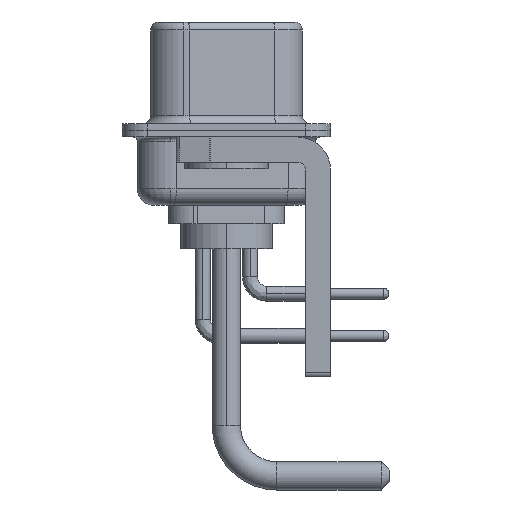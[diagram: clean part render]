
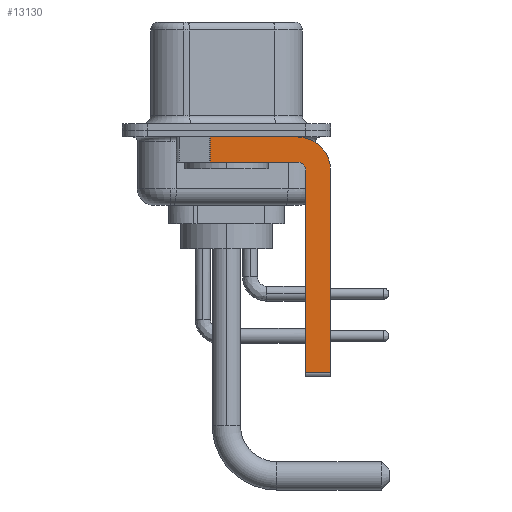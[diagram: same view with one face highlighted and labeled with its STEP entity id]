
A CAD part, left-side view. The second image highlights one B-rep face of the part: STEP entity #13130.
In plain terms, the highlighted planar face has unit normal (-1, 0, 0).
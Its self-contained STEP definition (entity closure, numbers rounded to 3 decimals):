
#246 = DIRECTION ( 'NONE',  ( 0., 0., -1. ) ) ;
#262 = EDGE_CURVE ( 'NONE', #14197, #24894, #24503, .T. ) ;
#716 = CARTESIAN_POINT ( 'NONE',  ( -2.9, -4.25, -2.4 ) ) ;
#851 = VERTEX_POINT ( 'NONE', #15234 ) ;
#991 = CIRCLE ( 'NONE', #23414, 0.5 ) ;
#1104 = CARTESIAN_POINT ( 'NONE',  ( -2.9, -4.25, -14.55 ) ) ;
#1154 = EDGE_CURVE ( 'NONE', #7924, #11928, #16393, .T. ) ;
#1262 = ORIENTED_EDGE ( 'NONE', *, *, #262, .F. ) ;
#1675 = CARTESIAN_POINT ( 'NONE',  ( -2.9, 0.978, -0.4 ) ) ;
#1800 = CIRCLE ( 'NONE', #5469, 2. ) ;
#2226 = CARTESIAN_POINT ( 'NONE',  ( -2.9, -4.25, -0.4 ) ) ;
#2501 = FACE_OUTER_BOUND ( 'NONE', #18995, .T. ) ;
#3681 = LINE ( 'NONE', #13634, #13141 ) ;
#4321 = DIRECTION ( 'NONE',  ( 1., 0., 0. ) ) ;
#4756 = CARTESIAN_POINT ( 'NONE',  ( -2.9, -6.25, -2.4 ) ) ;
#5011 = ORIENTED_EDGE ( 'NONE', *, *, #17259, .F. ) ;
#5469 = AXIS2_PLACEMENT_3D ( 'NONE', #20287, #4321, #18129 ) ;
#5486 = VERTEX_POINT ( 'NONE', #23102 ) ;
#5667 = CARTESIAN_POINT ( 'NONE',  ( -2.9, -4.25, -1.9 ) ) ;
#5718 = ORIENTED_EDGE ( 'NONE', *, *, #13471, .F. ) ;
#6594 = PLANE ( 'NONE',  #18527 ) ;
#7325 = VERTEX_POINT ( 'NONE', #8701 ) ;
#7575 = VERTEX_POINT ( 'NONE', #21443 ) ;
#7924 = VERTEX_POINT ( 'NONE', #23933 ) ;
#7932 = EDGE_CURVE ( 'NONE', #851, #7325, #12170, .T. ) ;
#8411 = VECTOR ( 'NONE', #23163, 1000. ) ;
#8622 = CARTESIAN_POINT ( 'NONE',  ( -2.9, -4.75, -14.8 ) ) ;
#8680 = DIRECTION ( 'NONE',  ( -1., 0., 0. ) ) ;
#8701 = CARTESIAN_POINT ( 'NONE',  ( -2.9, -4.75, -2.4 ) ) ;
#9018 = LINE ( 'NONE', #1104, #21106 ) ;
#9180 = ORIENTED_EDGE ( 'NONE', *, *, #10084, .T. ) ;
#9408 = VECTOR ( 'NONE', #16270, 1000. ) ;
#10084 = EDGE_CURVE ( 'NONE', #14197, #5486, #3681, .T. ) ;
#11452 = ORIENTED_EDGE ( 'NONE', *, *, #7932, .F. ) ;
#11636 = EDGE_CURVE ( 'NONE', #24894, #7924, #1800, .T. ) ;
#11928 = VERTEX_POINT ( 'NONE', #15655 ) ;
#12170 = LINE ( 'NONE', #8622, #9408 ) ;
#12856 = DIRECTION ( 'NONE',  ( 0., -1., 0. ) ) ;
#13126 = VECTOR ( 'NONE', #12856, 1000. ) ;
#13130 = ADVANCED_FACE ( 'NONE', ( #2501 ), #6594, .F. ) ;
#13141 = VECTOR ( 'NONE', #246, 1000. ) ;
#13471 = EDGE_CURVE ( 'NONE', #7575, #5486, #13690, .T. ) ;
#13634 = CARTESIAN_POINT ( 'NONE',  ( -2.9, 0.978, -1.9 ) ) ;
#13690 = LINE ( 'NONE', #5667, #8411 ) ;
#14197 = VERTEX_POINT ( 'NONE', #1675 ) ;
#14285 = DIRECTION ( 'NONE',  ( 0., 0., 1. ) ) ;
#14408 = CARTESIAN_POINT ( 'NONE',  ( -2.9, -4.25, -2.4 ) ) ;
#15067 = ORIENTED_EDGE ( 'NONE', *, *, #21968, .T. ) ;
#15234 = CARTESIAN_POINT ( 'NONE',  ( -2.9, -4.75, -14.55 ) ) ;
#15655 = CARTESIAN_POINT ( 'NONE',  ( -2.9, -6.25, -14.55 ) ) ;
#16024 = DIRECTION ( 'NONE',  ( 1., 0., 0. ) ) ;
#16270 = DIRECTION ( 'NONE',  ( 0., 0., 1. ) ) ;
#16300 = DIRECTION ( 'NONE',  ( 0., -1., 0. ) ) ;
#16393 = LINE ( 'NONE', #4756, #19032 ) ;
#17259 = EDGE_CURVE ( 'NONE', #7325, #7575, #991, .T. ) ;
#18011 = ORIENTED_EDGE ( 'NONE', *, *, #11636, .F. ) ;
#18129 = DIRECTION ( 'NONE',  ( 0., 0., -1. ) ) ;
#18527 = AXIS2_PLACEMENT_3D ( 'NONE', #716, #16024, #23821 ) ;
#18681 = DIRECTION ( 'NONE',  ( 0., 0., -1. ) ) ;
#18995 = EDGE_LOOP ( 'NONE', ( #1262, #9180, #5718, #5011, #11452, #15067, #23108, #18011 ) ) ;
#19032 = VECTOR ( 'NONE', #18681, 1000. ) ;
#20287 = CARTESIAN_POINT ( 'NONE',  ( -2.9, -4.25, -2.4 ) ) ;
#21106 = VECTOR ( 'NONE', #16300, 1000. ) ;
#21443 = CARTESIAN_POINT ( 'NONE',  ( -2.9, -4.25, -1.9 ) ) ;
#21968 = EDGE_CURVE ( 'NONE', #851, #11928, #9018, .T. ) ;
#22573 = CARTESIAN_POINT ( 'NONE',  ( -2.9, 3., -0.4 ) ) ;
#23102 = CARTESIAN_POINT ( 'NONE',  ( -2.9, 0.978, -1.9 ) ) ;
#23108 = ORIENTED_EDGE ( 'NONE', *, *, #1154, .F. ) ;
#23163 = DIRECTION ( 'NONE',  ( 0., 1., 0. ) ) ;
#23414 = AXIS2_PLACEMENT_3D ( 'NONE', #14408, #8680, #14285 ) ;
#23821 = DIRECTION ( 'NONE',  ( 0., 0., -1. ) ) ;
#23933 = CARTESIAN_POINT ( 'NONE',  ( -2.9, -6.25, -2.4 ) ) ;
#24503 = LINE ( 'NONE', #22573, #13126 ) ;
#24894 = VERTEX_POINT ( 'NONE', #2226 ) ;
